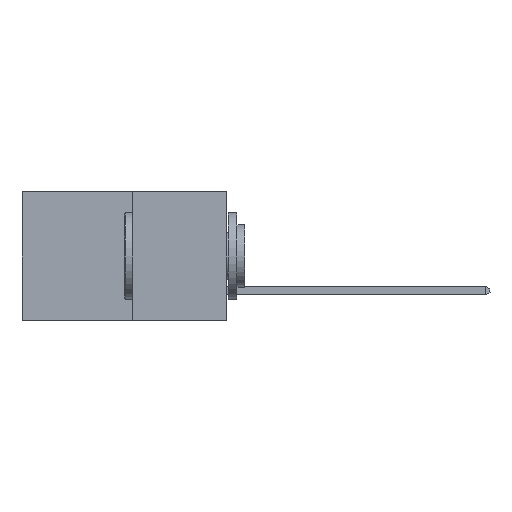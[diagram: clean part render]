
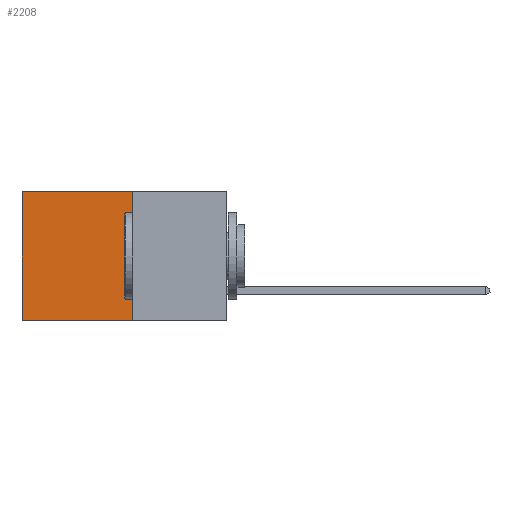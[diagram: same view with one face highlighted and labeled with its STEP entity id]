
A CAD part, left-side view. The second image highlights one B-rep face of the part: STEP entity #2208.
In plain terms, the highlighted planar face has unit normal (-1, 0, 0).
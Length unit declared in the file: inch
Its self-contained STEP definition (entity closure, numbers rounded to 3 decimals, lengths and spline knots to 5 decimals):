
#375 = LINE ( 'NONE', #8728, #2001 ) ;
#913 = VERTEX_POINT ( 'NONE', #7258 ) ;
#1219 = ORIENTED_EDGE ( 'NONE', *, *, #9287, .F. ) ;
#1268 = DIRECTION ( 'NONE',  ( 0., 0., -1. ) ) ;
#1339 = DIRECTION ( 'NONE',  ( 1., 0., 0. ) ) ;
#1381 = EDGE_CURVE ( 'NONE', #8984, #913, #4737, .T. ) ;
#1718 = ORIENTED_EDGE ( 'NONE', *, *, #6243, .T. ) ;
#2001 = VECTOR ( 'NONE', #4078, 39.37008 ) ;
#2150 = CARTESIAN_POINT ( 'NONE',  ( 0.277, 0.27, -0.37 ) ) ;
#2208 = ADVANCED_FACE ( 'NONE', ( #6279 ), #2375, .F. ) ;
#2375 = PLANE ( 'NONE',  #7365 ) ;
#2400 = DIRECTION ( 'NONE',  ( 0., 1., 0. ) ) ;
#2510 = DIRECTION ( 'NONE',  ( 0., 0., -1. ) ) ;
#3514 = LINE ( 'NONE', #2150, #5359 ) ;
#3538 = CARTESIAN_POINT ( 'NONE',  ( 0.277, 0.27, 0. ) ) ;
#4078 = DIRECTION ( 'NONE',  ( 0., 0., -1. ) ) ;
#4458 = VERTEX_POINT ( 'NONE', #3538 ) ;
#4737 = LINE ( 'NONE', #8006, #6762 ) ;
#5359 = VECTOR ( 'NONE', #2400, 39.37008 ) ;
#5384 = EDGE_LOOP ( 'NONE', ( #5541, #6263, #1219, #1718 ) ) ;
#5541 = ORIENTED_EDGE ( 'NONE', *, *, #1381, .T. ) ;
#6090 = CARTESIAN_POINT ( 'NONE',  ( 0.277, 0.59, 0. ) ) ;
#6243 = EDGE_CURVE ( 'NONE', #4458, #8984, #6937, .T. ) ;
#6263 = ORIENTED_EDGE ( 'NONE', *, *, #6614, .F. ) ;
#6279 = FACE_OUTER_BOUND ( 'NONE', #5384, .T. ) ;
#6595 = CARTESIAN_POINT ( 'NONE',  ( 0.277, 0.27, -0.37 ) ) ;
#6614 = EDGE_CURVE ( 'NONE', #9727, #913, #3514, .T. ) ;
#6762 = VECTOR ( 'NONE', #2510, 39.37008 ) ;
#6937 = LINE ( 'NONE', #7697, #8739 ) ;
#7258 = CARTESIAN_POINT ( 'NONE',  ( 0.277, 0.59, -0.37 ) ) ;
#7365 = AXIS2_PLACEMENT_3D ( 'NONE', #9363, #1339, #1268 ) ;
#7396 = DIRECTION ( 'NONE',  ( 0., 1., 0. ) ) ;
#7697 = CARTESIAN_POINT ( 'NONE',  ( 0.277, 0.27, 0. ) ) ;
#8006 = CARTESIAN_POINT ( 'NONE',  ( 0.277, 0.59, -0.37 ) ) ;
#8728 = CARTESIAN_POINT ( 'NONE',  ( 0.277, 0.27, -0.37 ) ) ;
#8739 = VECTOR ( 'NONE', #7396, 39.37008 ) ;
#8984 = VERTEX_POINT ( 'NONE', #6090 ) ;
#9287 = EDGE_CURVE ( 'NONE', #4458, #9727, #375, .T. ) ;
#9363 = CARTESIAN_POINT ( 'NONE',  ( 0.277, 0.27, -0.37 ) ) ;
#9727 = VERTEX_POINT ( 'NONE', #6595 ) ;
